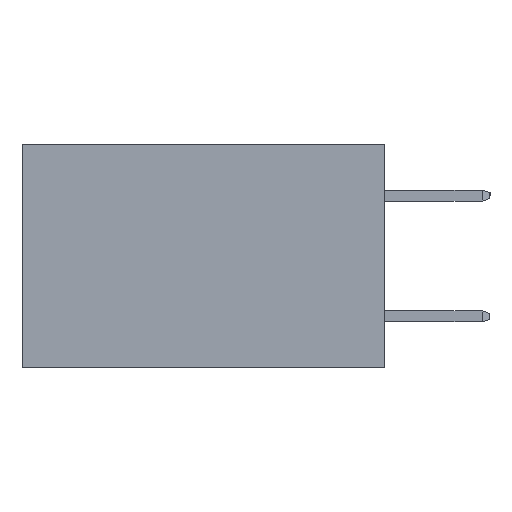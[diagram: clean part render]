
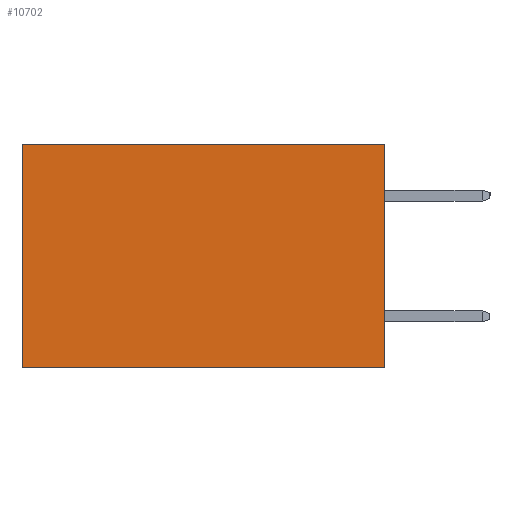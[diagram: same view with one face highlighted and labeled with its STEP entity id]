
A CAD part, left-side view. The second image highlights one B-rep face of the part: STEP entity #10702.
In plain terms, the highlighted planar face has unit normal (-1, 0, 0).
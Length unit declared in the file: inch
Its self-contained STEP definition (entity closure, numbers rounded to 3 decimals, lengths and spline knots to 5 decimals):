
#85 = ORIENTED_EDGE ( 'NONE', *, *, #5914, .F. ) ;
#1430 = EDGE_CURVE ( 'NONE', #7061, #10219, #4268, .T. ) ;
#1951 = CARTESIAN_POINT ( 'NONE',  ( 0.2615, 0.6, -0.37 ) ) ;
#2064 = CARTESIAN_POINT ( 'NONE',  ( 0.2615, 0., -0.37 ) ) ;
#2170 = DIRECTION ( 'NONE',  ( 0., 0., -1. ) ) ;
#2636 = ORIENTED_EDGE ( 'NONE', *, *, #7842, .T. ) ;
#3325 = DIRECTION ( 'NONE',  ( 0., 1., 0. ) ) ;
#3856 = DIRECTION ( 'NONE',  ( 0., 0., -1. ) ) ;
#4002 = DIRECTION ( 'NONE',  ( 0., 1., 0. ) ) ;
#4016 = CARTESIAN_POINT ( 'NONE',  ( 0.2615, 0., -0.37 ) ) ;
#4268 = LINE ( 'NONE', #7554, #9622 ) ;
#4697 = AXIS2_PLACEMENT_3D ( 'NONE', #7471, #9908, #2170 ) ;
#4945 = LINE ( 'NONE', #13964, #6226 ) ;
#5113 = VECTOR ( 'NONE', #13342, 39.37008 ) ;
#5320 = LINE ( 'NONE', #14120, #7171 ) ;
#5914 = EDGE_CURVE ( 'NONE', #14427, #11625, #5320, .T. ) ;
#6226 = VECTOR ( 'NONE', #3856, 39.37008 ) ;
#6342 = CARTESIAN_POINT ( 'NONE',  ( 0.2615, 0., 0. ) ) ;
#6461 = CARTESIAN_POINT ( 'NONE',  ( 0.2615, 0.6, 0. ) ) ;
#6610 = LINE ( 'NONE', #2064, #5113 ) ;
#7061 = VERTEX_POINT ( 'NONE', #6342 ) ;
#7171 = VECTOR ( 'NONE', #4002, 39.37008 ) ;
#7471 = CARTESIAN_POINT ( 'NONE',  ( 0.2615, 0., -0.37 ) ) ;
#7554 = CARTESIAN_POINT ( 'NONE',  ( 0.2615, 0., 0. ) ) ;
#7842 = EDGE_CURVE ( 'NONE', #10219, #11625, #4945, .T. ) ;
#7859 = ORIENTED_EDGE ( 'NONE', *, *, #1430, .T. ) ;
#8514 = FACE_OUTER_BOUND ( 'NONE', #14163, .T. ) ;
#9622 = VECTOR ( 'NONE', #3325, 39.37008 ) ;
#9735 = EDGE_CURVE ( 'NONE', #7061, #14427, #6610, .T. ) ;
#9908 = DIRECTION ( 'NONE',  ( 1., 0., 0. ) ) ;
#10219 = VERTEX_POINT ( 'NONE', #6461 ) ;
#10702 = ADVANCED_FACE ( 'NONE', ( #8514 ), #14369, .F. ) ;
#11625 = VERTEX_POINT ( 'NONE', #1951 ) ;
#13342 = DIRECTION ( 'NONE',  ( 0., 0., -1. ) ) ;
#13688 = ORIENTED_EDGE ( 'NONE', *, *, #9735, .F. ) ;
#13964 = CARTESIAN_POINT ( 'NONE',  ( 0.2615, 0.6, -0.37 ) ) ;
#14120 = CARTESIAN_POINT ( 'NONE',  ( 0.2615, 0., -0.37 ) ) ;
#14163 = EDGE_LOOP ( 'NONE', ( #2636, #85, #13688, #7859 ) ) ;
#14369 = PLANE ( 'NONE',  #4697 ) ;
#14427 = VERTEX_POINT ( 'NONE', #4016 ) ;
